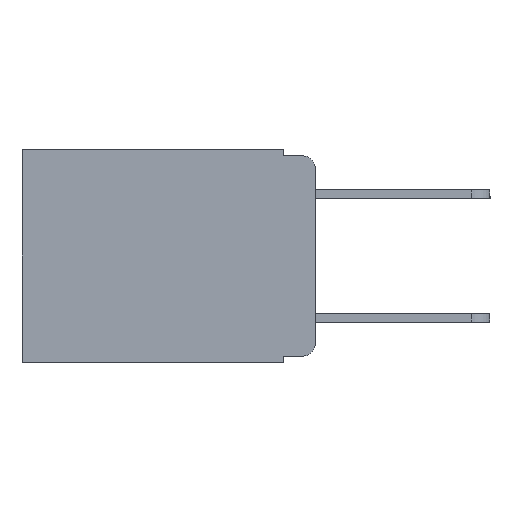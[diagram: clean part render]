
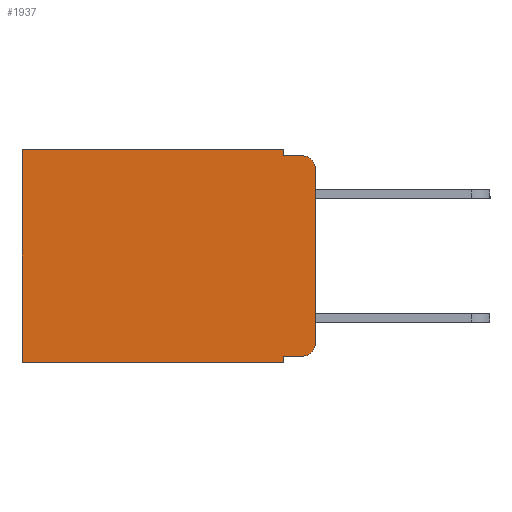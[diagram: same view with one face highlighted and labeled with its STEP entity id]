
A CAD part, left-side view. The second image highlights one B-rep face of the part: STEP entity #1937.
In plain terms, the highlighted planar face has unit normal (-1, 0, 0).
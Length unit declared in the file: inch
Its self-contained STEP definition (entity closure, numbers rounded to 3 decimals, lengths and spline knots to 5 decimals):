
#124 = ORIENTED_EDGE ( 'NONE', *, *, #13867, .F. ) ;
#246 = LINE ( 'NONE', #14976, #15417 ) ;
#287 = VERTEX_POINT ( 'NONE', #9703 ) ;
#296 = CARTESIAN_POINT ( 'NONE',  ( 0.298, 0., 0. ) ) ;
#302 = VECTOR ( 'NONE', #3346, 39.37008 ) ;
#340 = ORIENTED_EDGE ( 'NONE', *, *, #11529, .T. ) ;
#477 = CIRCLE ( 'NONE', #1756, 0.02 ) ;
#479 = CARTESIAN_POINT ( 'NONE',  ( 0.298, 0.051, 0. ) ) ;
#530 = ORIENTED_EDGE ( 'NONE', *, *, #15635, .T. ) ;
#671 = VECTOR ( 'NONE', #8203, 39.37008 ) ;
#840 = LINE ( 'NONE', #15321, #15509 ) ;
#1018 = EDGE_CURVE ( 'NONE', #14783, #12434, #7373, .T. ) ;
#1186 = LINE ( 'NONE', #11078, #671 ) ;
#1756 = AXIS2_PLACEMENT_3D ( 'NONE', #16679, #8577, #17957 ) ;
#1937 = ADVANCED_FACE ( 'NONE', ( #11599 ), #5396, .F. ) ;
#1992 = VERTEX_POINT ( 'NONE', #10887 ) ;
#2274 = AXIS2_PLACEMENT_3D ( 'NONE', #296, #14544, #14567 ) ;
#2581 = EDGE_LOOP ( 'NONE', ( #10914, #340, #12586, #12992, #9361, #10930, #4998, #124, #530, #17953 ) ) ;
#3069 = VERTEX_POINT ( 'NONE', #16762 ) ;
#3095 = DIRECTION ( 'NONE',  ( 0., 1., 0. ) ) ;
#3148 = EDGE_CURVE ( 'NONE', #3069, #287, #840, .T. ) ;
#3346 = DIRECTION ( 'NONE',  ( 0., -1., 0. ) ) ;
#3747 = VERTEX_POINT ( 'NONE', #14176 ) ;
#3970 = VECTOR ( 'NONE', #9309, 39.37008 ) ;
#4381 = LINE ( 'NONE', #7604, #302 ) ;
#4489 = CARTESIAN_POINT ( 'NONE',  ( 0.298, 0.473, 0. ) ) ;
#4853 = DIRECTION ( 'NONE',  ( 0., 0., -1. ) ) ;
#4998 = ORIENTED_EDGE ( 'NONE', *, *, #3148, .F. ) ;
#5302 = VECTOR ( 'NONE', #18084, 39.37008 ) ;
#5396 = PLANE ( 'NONE',  #2274 ) ;
#5784 = EDGE_CURVE ( 'NONE', #11916, #12434, #246, .T. ) ;
#5964 = VERTEX_POINT ( 'NONE', #14609 ) ;
#6734 = VERTEX_POINT ( 'NONE', #4489 ) ;
#6922 = EDGE_CURVE ( 'NONE', #3747, #6734, #16805, .T. ) ;
#7373 = CIRCLE ( 'NONE', #18177, 0.02 ) ;
#7604 = CARTESIAN_POINT ( 'NONE',  ( 0.298, 0.051, -0.333 ) ) ;
#7691 = DIRECTION ( 'NONE',  ( 0., 0., -1. ) ) ;
#7927 = VERTEX_POINT ( 'NONE', #15111 ) ;
#8138 = CARTESIAN_POINT ( 'NONE',  ( 0.298, 0., -0.313 ) ) ;
#8203 = DIRECTION ( 'NONE',  ( 0., -1., 0. ) ) ;
#8222 = CARTESIAN_POINT ( 'NONE',  ( 0.298, 0., -0.03 ) ) ;
#8577 = DIRECTION ( 'NONE',  ( -1., 0., 0. ) ) ;
#9309 = DIRECTION ( 'NONE',  ( 0., 0., -1. ) ) ;
#9361 = ORIENTED_EDGE ( 'NONE', *, *, #6922, .T. ) ;
#9703 = CARTESIAN_POINT ( 'NONE',  ( 0.298, 0.473, -0.343 ) ) ;
#10687 = CARTESIAN_POINT ( 'NONE',  ( 0.298, 0., 0. ) ) ;
#10751 = CARTESIAN_POINT ( 'NONE',  ( 0.298, 0.02, -0.313 ) ) ;
#10887 = CARTESIAN_POINT ( 'NONE',  ( 0.298, 0.051, -0.333 ) ) ;
#10914 = ORIENTED_EDGE ( 'NONE', *, *, #5784, .F. ) ;
#10930 = ORIENTED_EDGE ( 'NONE', *, *, #15051, .T. ) ;
#11078 = CARTESIAN_POINT ( 'NONE',  ( 0.298, 0.051, -0.01 ) ) ;
#11329 = VECTOR ( 'NONE', #7691, 39.37008 ) ;
#11529 = EDGE_CURVE ( 'NONE', #11916, #5964, #477, .T. ) ;
#11599 = FACE_OUTER_BOUND ( 'NONE', #2581, .T. ) ;
#11916 = VERTEX_POINT ( 'NONE', #8222 ) ;
#12040 = LINE ( 'NONE', #479, #3970 ) ;
#12434 = VERTEX_POINT ( 'NONE', #8138 ) ;
#12452 = EDGE_CURVE ( 'NONE', #7927, #5964, #1186, .T. ) ;
#12586 = ORIENTED_EDGE ( 'NONE', *, *, #12452, .F. ) ;
#12992 = ORIENTED_EDGE ( 'NONE', *, *, #14184, .F. ) ;
#13328 = VECTOR ( 'NONE', #17401, 39.37008 ) ;
#13867 = EDGE_CURVE ( 'NONE', #1992, #3069, #12040, .T. ) ;
#14176 = CARTESIAN_POINT ( 'NONE',  ( 0.298, 0.051, 0. ) ) ;
#14184 = EDGE_CURVE ( 'NONE', #3747, #7927, #16739, .T. ) ;
#14544 = DIRECTION ( 'NONE',  ( 1., 0., 0. ) ) ;
#14567 = DIRECTION ( 'NONE',  ( 0., 0., -1. ) ) ;
#14609 = CARTESIAN_POINT ( 'NONE',  ( 0.298, 0.02, -0.01 ) ) ;
#14783 = VERTEX_POINT ( 'NONE', #16656 ) ;
#14864 = LINE ( 'NONE', #15942, #11329 ) ;
#14976 = CARTESIAN_POINT ( 'NONE',  ( 0.298, 0., 0. ) ) ;
#14990 = DIRECTION ( 'NONE',  ( 0., 0., -1. ) ) ;
#15051 = EDGE_CURVE ( 'NONE', #6734, #287, #14864, .T. ) ;
#15111 = CARTESIAN_POINT ( 'NONE',  ( 0.298, 0.051, -0.01 ) ) ;
#15321 = CARTESIAN_POINT ( 'NONE',  ( 0.298, 0., -0.343 ) ) ;
#15417 = VECTOR ( 'NONE', #4853, 39.37008 ) ;
#15509 = VECTOR ( 'NONE', #3095, 39.37008 ) ;
#15635 = EDGE_CURVE ( 'NONE', #1992, #14783, #4381, .T. ) ;
#15942 = CARTESIAN_POINT ( 'NONE',  ( 0.298, 0.473, 0. ) ) ;
#16656 = CARTESIAN_POINT ( 'NONE',  ( 0.298, 0.02, -0.333 ) ) ;
#16679 = CARTESIAN_POINT ( 'NONE',  ( 0.298, 0.02, -0.03 ) ) ;
#16739 = LINE ( 'NONE', #18023, #5302 ) ;
#16762 = CARTESIAN_POINT ( 'NONE',  ( 0.298, 0.051, -0.343 ) ) ;
#16805 = LINE ( 'NONE', #10687, #13328 ) ;
#17401 = DIRECTION ( 'NONE',  ( 0., 1., 0. ) ) ;
#17953 = ORIENTED_EDGE ( 'NONE', *, *, #1018, .T. ) ;
#17957 = DIRECTION ( 'NONE',  ( 0., 0., -1. ) ) ;
#18023 = CARTESIAN_POINT ( 'NONE',  ( 0.298, 0.051, 0. ) ) ;
#18084 = DIRECTION ( 'NONE',  ( 0., 0., -1. ) ) ;
#18119 = DIRECTION ( 'NONE',  ( -1., 0., 0. ) ) ;
#18177 = AXIS2_PLACEMENT_3D ( 'NONE', #10751, #18119, #14990 ) ;
